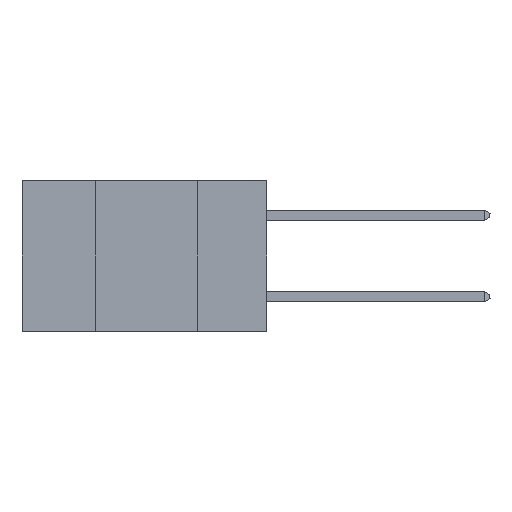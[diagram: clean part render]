
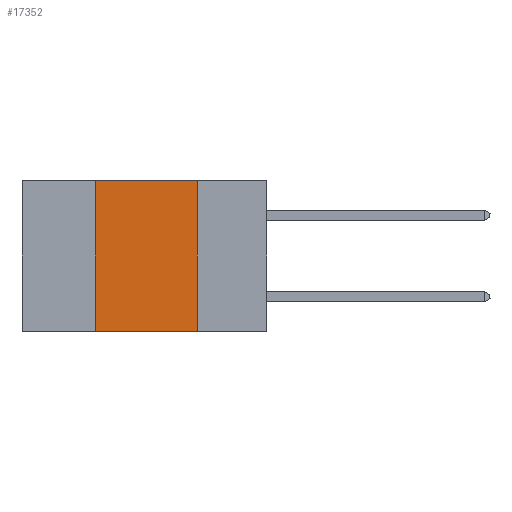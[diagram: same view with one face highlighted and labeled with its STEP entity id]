
A CAD part, left-side view. The second image highlights one B-rep face of the part: STEP entity #17352.
In plain terms, the highlighted planar face has unit normal (-1, 0, 0).
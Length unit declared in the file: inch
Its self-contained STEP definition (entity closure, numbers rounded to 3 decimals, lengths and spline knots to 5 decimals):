
#465 = VERTEX_POINT ( 'NONE', #20027 ) ;
#1077 = VECTOR ( 'NONE', #30948, 39.37008 ) ;
#3680 = VECTOR ( 'NONE', #12440, 39.37008 ) ;
#3807 = CARTESIAN_POINT ( 'NONE',  ( 0., 0.17, 0. ) ) ;
#5706 = LINE ( 'NONE', #14613, #13047 ) ;
#6236 = CARTESIAN_POINT ( 'NONE',  ( 0., 0.17, -0.37 ) ) ;
#7289 = DIRECTION ( 'NONE',  ( 0., 0., -1. ) ) ;
#7298 = ORIENTED_EDGE ( 'NONE', *, *, #28573, .F. ) ;
#9653 = PLANE ( 'NONE',  #19101 ) ;
#10170 = CARTESIAN_POINT ( 'NONE',  ( 0., 0.42, 0. ) ) ;
#11290 = ORIENTED_EDGE ( 'NONE', *, *, #13426, .F. ) ;
#11336 = LINE ( 'NONE', #10170, #3680 ) ;
#11660 = DIRECTION ( 'NONE',  ( 0., -1., 0. ) ) ;
#12440 = DIRECTION ( 'NONE',  ( 0., 0., 1. ) ) ;
#13047 = VECTOR ( 'NONE', #14723, 39.37008 ) ;
#13426 = EDGE_CURVE ( 'NONE', #22065, #23729, #5706, .T. ) ;
#14498 = CARTESIAN_POINT ( 'NONE',  ( 0., 0.42, 0. ) ) ;
#14613 = CARTESIAN_POINT ( 'NONE',  ( 0., 0.6, 0. ) ) ;
#14723 = DIRECTION ( 'NONE',  ( 0., -1., 0. ) ) ;
#14839 = EDGE_CURVE ( 'NONE', #465, #30581, #27923, .T. ) ;
#15171 = ORIENTED_EDGE ( 'NONE', *, *, #14839, .T. ) ;
#17352 = ADVANCED_FACE ( 'NONE', ( #28924 ), #9653, .F. ) ;
#19101 = AXIS2_PLACEMENT_3D ( 'NONE', #24277, #19448, #7289 ) ;
#19448 = DIRECTION ( 'NONE',  ( 1., 0., 0. ) ) ;
#20027 = CARTESIAN_POINT ( 'NONE',  ( 0., 0.42, -0.37 ) ) ;
#21071 = LINE ( 'NONE', #28810, #1077 ) ;
#22065 = VERTEX_POINT ( 'NONE', #14498 ) ;
#23729 = VERTEX_POINT ( 'NONE', #3807 ) ;
#24277 = CARTESIAN_POINT ( 'NONE',  ( 0., 0.6, 0. ) ) ;
#26162 = CARTESIAN_POINT ( 'NONE',  ( 0., 0.6, -0.37 ) ) ;
#27886 = ORIENTED_EDGE ( 'NONE', *, *, #30667, .F. ) ;
#27923 = LINE ( 'NONE', #26162, #30252 ) ;
#28278 = EDGE_LOOP ( 'NONE', ( #27886, #11290, #7298, #15171 ) ) ;
#28573 = EDGE_CURVE ( 'NONE', #465, #22065, #11336, .T. ) ;
#28810 = CARTESIAN_POINT ( 'NONE',  ( 0., 0.17, 0. ) ) ;
#28924 = FACE_OUTER_BOUND ( 'NONE', #28278, .T. ) ;
#30252 = VECTOR ( 'NONE', #11660, 39.37008 ) ;
#30581 = VERTEX_POINT ( 'NONE', #6236 ) ;
#30667 = EDGE_CURVE ( 'NONE', #23729, #30581, #21071, .T. ) ;
#30948 = DIRECTION ( 'NONE',  ( 0., 0., -1. ) ) ;
